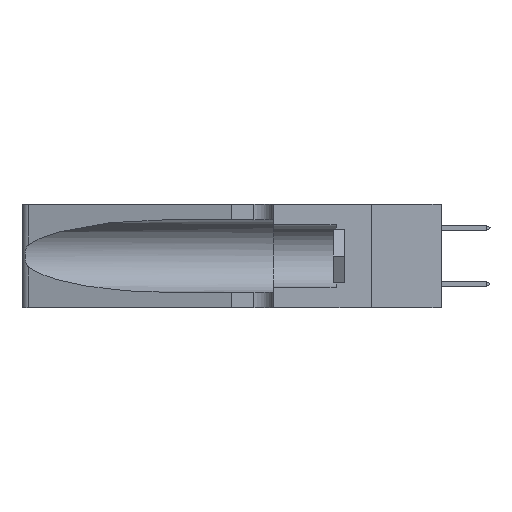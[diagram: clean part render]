
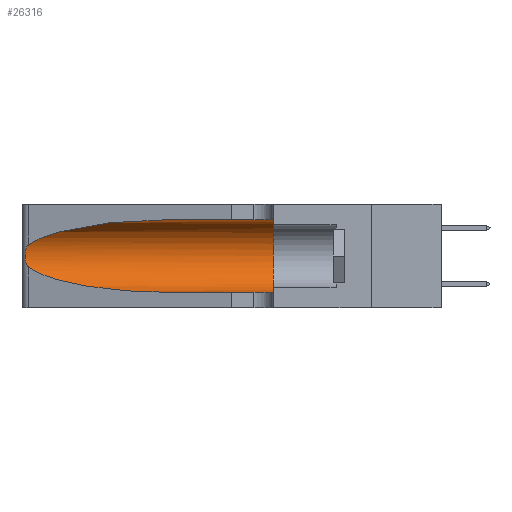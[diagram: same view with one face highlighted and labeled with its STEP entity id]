
A CAD part, left-side view. The second image highlights one B-rep face of the part: STEP entity #26316.
In plain terms, the highlighted cylindrical face has radius 3.308 mm (diameter 6.617 mm), a partial arc.
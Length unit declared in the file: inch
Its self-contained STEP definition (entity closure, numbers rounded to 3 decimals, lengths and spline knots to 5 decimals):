
#1383 = EDGE_CURVE ( 'NONE', #12562, #26134, #7757, .T. ) ;
#1422 = EDGE_CURVE ( 'NONE', #26134, #12942, #2190, .T. ) ;
#1689 = ORIENTED_EDGE ( 'NONE', *, *, #19041, .F. ) ;
#2190 = LINE ( 'NONE', #8306, #14545 ) ;
#2390 = CARTESIAN_POINT ( 'NONE',  ( 0.25487, 1.22718, 0.22369 ) ) ;
#2503 = CARTESIAN_POINT ( 'NONE',  ( 0.25487, 1.22718, 0.14631 ) ) ;
#2847 = CARTESIAN_POINT ( 'NONE',  ( 0.25487, 1.22718, 0.22369 ) ) ;
#5016 = CARTESIAN_POINT ( 'NONE',  ( 0.25639, 1.23184, 0.21858 ) ) ;
#5101 = VERTEX_POINT ( 'NONE', #16220 ) ;
#5250 = CARTESIAN_POINT ( 'NONE',  ( 0.1305, 0.35, 0.31525 ) ) ;
#5314 = FACE_OUTER_BOUND ( 'NONE', #11050, .T. ) ;
#5549 = CARTESIAN_POINT ( 'NONE',  ( 0.2373, 1.15595, 0.08982 ) ) ;
#5780 = DIRECTION ( 'NONE',  ( 0., -1., 0. ) ) ;
#7679 = CARTESIAN_POINT ( 'NONE',  ( 0.25854, 1.2359, 0.20912 ) ) ;
#7757 =( BOUNDED_CURVE ( )  B_SPLINE_CURVE ( 3, ( #13521, #5549, #29225, #31853 ),
 .UNSPECIFIED., .F., .T. ) 
 B_SPLINE_CURVE_WITH_KNOTS ( ( 4, 4 ),
 ( 3.44316, 4.71239 ),
 .UNSPECIFIED. ) 
 CURVE ( )  GEOMETRIC_REPRESENTATION_ITEM ( )  RATIONAL_B_SPLINE_CURVE ( ( 1., 0.87, 0.87, 1. ) ) 
 REPRESENTATION_ITEM ( '' )  );
#8020 = LINE ( 'NONE', #27128, #20382 ) ;
#8028 = EDGE_CURVE ( 'NONE', #5101, #23810, #11334, .T. ) ;
#8087 = CARTESIAN_POINT ( 'NONE',  ( 0.1305, 0.35, 0.185 ) ) ;
#8306 = CARTESIAN_POINT ( 'NONE',  ( 0.1305, 1.61858, 0.05475 ) ) ;
#9849 = CARTESIAN_POINT ( 'NONE',  ( 0.1305, 0.72297, 0.05475 ) ) ;
#9972 = VERTEX_POINT ( 'NONE', #5250 ) ;
#10320 = CARTESIAN_POINT ( 'NONE',  ( 0.26075, 1.23896, 0.19203 ) ) ;
#10528 = DIRECTION ( 'NONE',  ( 0., 0., -1. ) ) ;
#10530 = ORIENTED_EDGE ( 'NONE', *, *, #8028, .T. ) ;
#10606 = ORIENTED_EDGE ( 'NONE', *, *, #13755, .F. ) ;
#10736 = DIRECTION ( 'NONE',  ( 0., 0., 1. ) ) ;
#11050 = EDGE_LOOP ( 'NONE', ( #10530, #17138, #17433, #23221, #1689, #10606 ) ) ;
#11227 = AXIS2_PLACEMENT_3D ( 'NONE', #8087, #26489, #10736 ) ;
#11334 =( BOUNDED_CURVE ( )  B_SPLINE_CURVE ( 3, ( #23762, #13342, #18619, #2847 ),
 .UNSPECIFIED., .F., .T. ) 
 B_SPLINE_CURVE_WITH_KNOTS ( ( 4, 4 ),
 ( 1.5708, 2.84003 ),
 .UNSPECIFIED. ) 
 CURVE ( )  GEOMETRIC_REPRESENTATION_ITEM ( )  RATIONAL_B_SPLINE_CURVE ( ( 1., 0.87, 0.87, 1. ) ) 
 REPRESENTATION_ITEM ( '' )  );
#12562 = VERTEX_POINT ( 'NONE', #33245 ) ;
#12942 = VERTEX_POINT ( 'NONE', #29436 ) ;
#12989 = CARTESIAN_POINT ( 'NONE',  ( 0.26017, 1.23833, 0.17102 ) ) ;
#13342 = CARTESIAN_POINT ( 'NONE',  ( 0.18966, 0.96281, 0.31525 ) ) ;
#13497 = CARTESIAN_POINT ( 'NONE',  ( 0.25487, 1.22718, 0.22369 ) ) ;
#13521 = CARTESIAN_POINT ( 'NONE',  ( 0.25487, 1.22718, 0.14631 ) ) ;
#13755 = EDGE_CURVE ( 'NONE', #5101, #9972, #8020, .T. ) ;
#14022 = CIRCLE ( 'NONE', #11227, 0.13025 ) ;
#14049 = DIRECTION ( 'NONE',  ( 0., -1., 0. ) ) ;
#14545 = VECTOR ( 'NONE', #5780, 39.37008 ) ;
#15604 = CARTESIAN_POINT ( 'NONE',  ( 0.25789, 1.23486, 0.15765 ) ) ;
#16220 = CARTESIAN_POINT ( 'NONE',  ( 0.1305, 0.72297, 0.31525 ) ) ;
#17138 = ORIENTED_EDGE ( 'NONE', *, *, #24252, .T. ) ;
#17433 = ORIENTED_EDGE ( 'NONE', *, *, #1383, .T. ) ;
#17690 = CYLINDRICAL_SURFACE ( 'NONE', #22620, 0.13025 ) ;
#18154 = CARTESIAN_POINT ( 'NONE',  ( 0.25555, 1.22994, 0.2215 ) ) ;
#18257 = CARTESIAN_POINT ( 'NONE',  ( 0.25555, 1.22993, 0.14849 ) ) ;
#18619 = CARTESIAN_POINT ( 'NONE',  ( 0.2373, 1.15595, 0.28018 ) ) ;
#19041 = EDGE_CURVE ( 'NONE', #9972, #12942, #14022, .T. ) ;
#20382 = VECTOR ( 'NONE', #14049, 39.37008 ) ;
#22620 = AXIS2_PLACEMENT_3D ( 'NONE', #26282, #23621, #10528 ) ;
#23221 = ORIENTED_EDGE ( 'NONE', *, *, #1422, .T. ) ;
#23410 = CARTESIAN_POINT ( 'NONE',  ( 0.25787, 1.23484, 0.2124 ) ) ;
#23621 = DIRECTION ( 'NONE',  ( 0., -1., 0. ) ) ;
#23762 = CARTESIAN_POINT ( 'NONE',  ( 0.1305, 0.72297, 0.31525 ) ) ;
#23810 = VERTEX_POINT ( 'NONE', #13497 ) ;
#24252 = EDGE_CURVE ( 'NONE', #23810, #12562, #30696, .T. ) ;
#26062 = CARTESIAN_POINT ( 'NONE',  ( 0.26018, 1.23835, 0.19895 ) ) ;
#26134 = VERTEX_POINT ( 'NONE', #9849 ) ;
#26282 = CARTESIAN_POINT ( 'NONE',  ( 0.1305, 1.61858, 0.185 ) ) ;
#26316 = ADVANCED_FACE ( 'NONE', ( #5314 ), #17690, .F. ) ;
#26489 = DIRECTION ( 'NONE',  ( 0., 1., 0. ) ) ;
#27128 = CARTESIAN_POINT ( 'NONE',  ( 0.1305, 1.61858, 0.31525 ) ) ;
#28690 = CARTESIAN_POINT ( 'NONE',  ( 0.26075, 1.23896, 0.178 ) ) ;
#29225 = CARTESIAN_POINT ( 'NONE',  ( 0.18966, 0.96281, 0.05475 ) ) ;
#29436 = CARTESIAN_POINT ( 'NONE',  ( 0.1305, 0.35, 0.05475 ) ) ;
#30696 = B_SPLINE_CURVE_WITH_KNOTS ( 'NONE', 3,
 ( #2390, #18154, #5016, #23410, #7679, #26062, #10320, #28690, #12989, #31329, #15604, #33930, #18257, #2503 ),
 .UNSPECIFIED., .F., .F.,
 ( 4, 2, 2, 2, 2, 2, 4 ),
 ( 0., 0.00027, 0.00053, 0.00107, 0.0016, 0.00187, 0.00214 ),
 .UNSPECIFIED. ) ;
#31329 = CARTESIAN_POINT ( 'NONE',  ( 0.25856, 1.23593, 0.16098 ) ) ;
#31853 = CARTESIAN_POINT ( 'NONE',  ( 0.1305, 0.72297, 0.05475 ) ) ;
#33245 = CARTESIAN_POINT ( 'NONE',  ( 0.25487, 1.22718, 0.14631 ) ) ;
#33930 = CARTESIAN_POINT ( 'NONE',  ( 0.25639, 1.23186, 0.15144 ) ) ;
